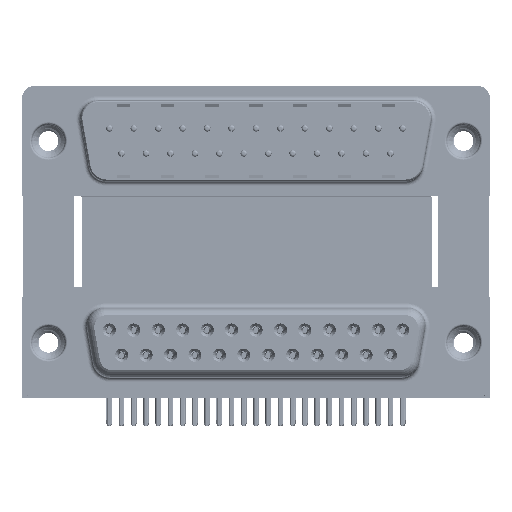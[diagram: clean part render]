
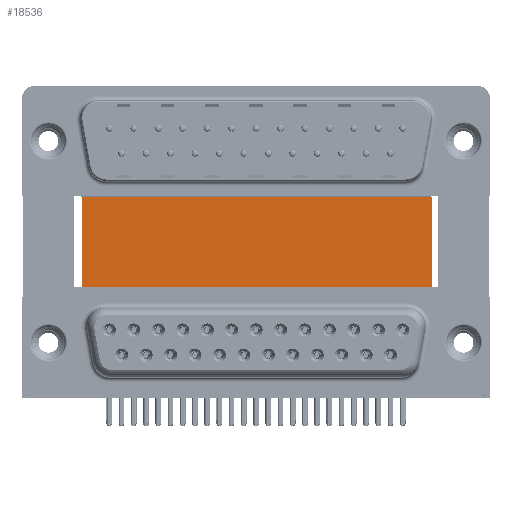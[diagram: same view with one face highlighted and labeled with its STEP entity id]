
A CAD part, top view. The second image highlights one B-rep face of the part: STEP entity #18536.
In plain terms, the highlighted planar face has unit normal (0, 0, 1).
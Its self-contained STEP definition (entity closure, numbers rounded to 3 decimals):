
#1542 = DIRECTION ( 'NONE',  ( -1., 0., 0. ) ) ;
#3378 = VECTOR ( 'NONE', #47136, 1000. ) ;
#3862 = VECTOR ( 'NONE', #48435, 1000. ) ;
#3957 = EDGE_CURVE ( 'NONE', #18774, #43946, #39143, .T. ) ;
#4873 = PLANE ( 'NONE',  #36631 ) ;
#9331 = CARTESIAN_POINT ( 'NONE',  ( 43.43, 16.585, -12. ) ) ;
#10310 = ORIENTED_EDGE ( 'NONE', *, *, #37071, .F. ) ;
#11086 = VERTEX_POINT ( 'NONE', #22036 ) ;
#15130 = LINE ( 'NONE', #52334, #3862 ) ;
#15546 = VECTOR ( 'NONE', #21247, 1000. ) ;
#17637 = FACE_OUTER_BOUND ( 'NONE', #39056, .T. ) ;
#18084 = CARTESIAN_POINT ( 'NONE',  ( 3.79, 16.585, -12. ) ) ;
#18536 = ADVANCED_FACE ( 'NONE', ( #17637 ), #4873, .F. ) ;
#18774 = VERTEX_POINT ( 'NONE', #18084 ) ;
#19603 = ORIENTED_EDGE ( 'NONE', *, *, #30156, .T. ) ;
#21018 = EDGE_CURVE ( 'NONE', #52029, #11086, #50949, .T. ) ;
#21247 = DIRECTION ( 'NONE',  ( 0., -1., 0. ) ) ;
#22036 = CARTESIAN_POINT ( 'NONE',  ( 43.43, -3.735, -12. ) ) ;
#22576 = CARTESIAN_POINT ( 'NONE',  ( 3.79, 16.585, -12. ) ) ;
#23227 = CARTESIAN_POINT ( 'NONE',  ( 3.79, -3.735, -12. ) ) ;
#25064 = VECTOR ( 'NONE', #30263, 1000. ) ;
#25747 = LINE ( 'NONE', #37991, #3378 ) ;
#26076 = CARTESIAN_POINT ( 'NONE',  ( 3.79, 16.585, -12. ) ) ;
#30156 = EDGE_CURVE ( 'NONE', #43946, #11086, #15130, .T. ) ;
#30263 = DIRECTION ( 'NONE',  ( 0., -1., 0. ) ) ;
#30679 = ORIENTED_EDGE ( 'NONE', *, *, #3957, .T. ) ;
#36631 = AXIS2_PLACEMENT_3D ( 'NONE', #22576, #39525, #1542 ) ;
#37071 = EDGE_CURVE ( 'NONE', #18774, #52029, #25747, .T. ) ;
#37991 = CARTESIAN_POINT ( 'NONE',  ( 3.79, 16.585, -12. ) ) ;
#39056 = EDGE_LOOP ( 'NONE', ( #19603, #53144, #10310, #30679 ) ) ;
#39143 = LINE ( 'NONE', #26076, #25064 ) ;
#39525 = DIRECTION ( 'NONE',  ( 0., 0., -1. ) ) ;
#42554 = CARTESIAN_POINT ( 'NONE',  ( 43.43, 16.585, -12. ) ) ;
#43946 = VERTEX_POINT ( 'NONE', #23227 ) ;
#47136 = DIRECTION ( 'NONE',  ( 1., 0., 0. ) ) ;
#48435 = DIRECTION ( 'NONE',  ( 1., 0., 0. ) ) ;
#50949 = LINE ( 'NONE', #9331, #15546 ) ;
#52029 = VERTEX_POINT ( 'NONE', #42554 ) ;
#52334 = CARTESIAN_POINT ( 'NONE',  ( 3.79, -3.735, -12. ) ) ;
#53144 = ORIENTED_EDGE ( 'NONE', *, *, #21018, .F. ) ;
